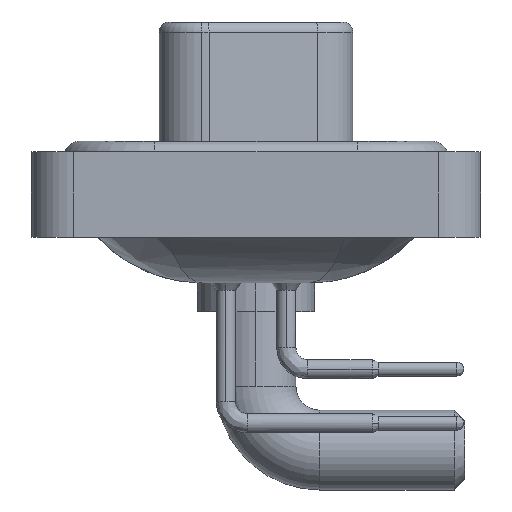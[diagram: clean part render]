
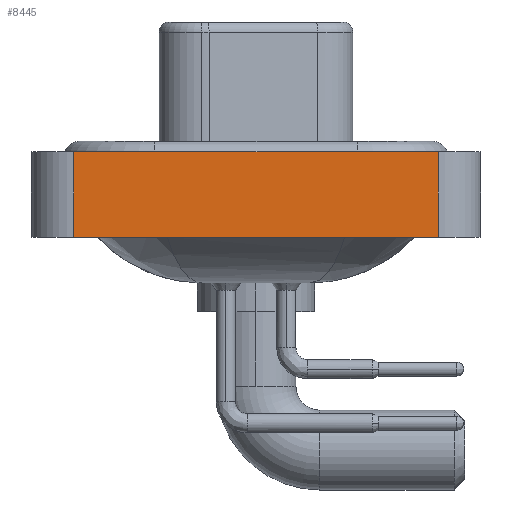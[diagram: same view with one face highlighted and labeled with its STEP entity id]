
A CAD part, left-side view. The second image highlights one B-rep face of the part: STEP entity #8445.
In plain terms, the highlighted planar face has unit normal (-1, 0, 0).
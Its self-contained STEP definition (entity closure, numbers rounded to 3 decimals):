
#60 = CARTESIAN_POINT ( 'NONE',  ( -7.25, 8.55, 0.4 ) ) ;
#461 = VERTEX_POINT ( 'NONE', #8579 ) ;
#969 = CARTESIAN_POINT ( 'NONE',  ( -7.25, -8.55, -3.6 ) ) ;
#2506 = EDGE_LOOP ( 'NONE', ( #13287, #8062, #5538, #6797 ) ) ;
#2616 = VECTOR ( 'NONE', #13395, 1000. ) ;
#3873 = LINE ( 'NONE', #14278, #11997 ) ;
#5166 = FACE_OUTER_BOUND ( 'NONE', #2506, .T. ) ;
#5538 = ORIENTED_EDGE ( 'NONE', *, *, #8697, .F. ) ;
#6797 = ORIENTED_EDGE ( 'NONE', *, *, #21317, .T. ) ;
#7086 = CARTESIAN_POINT ( 'NONE',  ( -7.25, 8.55, -3.6 ) ) ;
#7557 = DIRECTION ( 'NONE',  ( 0., -1., 0. ) ) ;
#8062 = ORIENTED_EDGE ( 'NONE', *, *, #9847, .F. ) ;
#8277 = DIRECTION ( 'NONE',  ( 0., 0., 1. ) ) ;
#8313 = VECTOR ( 'NONE', #21880, 1000. ) ;
#8445 = ADVANCED_FACE ( 'NONE', ( #5166 ), #14073, .T. ) ;
#8579 = CARTESIAN_POINT ( 'NONE',  ( -7.25, -8.55, 0.4 ) ) ;
#8697 = EDGE_CURVE ( 'NONE', #20557, #12375, #11163, .T. ) ;
#9431 = CARTESIAN_POINT ( 'NONE',  ( -7.25, 8.55, -3.6 ) ) ;
#9593 = AXIS2_PLACEMENT_3D ( 'NONE', #21110, #10588, #8277 ) ;
#9847 = EDGE_CURVE ( 'NONE', #12375, #461, #3873, .T. ) ;
#9947 = EDGE_CURVE ( 'NONE', #16285, #461, #20246, .T. ) ;
#10588 = DIRECTION ( 'NONE',  ( -1., 0., 0. ) ) ;
#11163 = LINE ( 'NONE', #9431, #13009 ) ;
#11997 = VECTOR ( 'NONE', #7557, 1000. ) ;
#12375 = VERTEX_POINT ( 'NONE', #60 ) ;
#13009 = VECTOR ( 'NONE', #16471, 1000. ) ;
#13287 = ORIENTED_EDGE ( 'NONE', *, *, #9947, .T. ) ;
#13395 = DIRECTION ( 'NONE',  ( 0., -1., 0. ) ) ;
#14073 = PLANE ( 'NONE',  #9593 ) ;
#14278 = CARTESIAN_POINT ( 'NONE',  ( -7.25, -8.55, 0.4 ) ) ;
#16285 = VERTEX_POINT ( 'NONE', #18890 ) ;
#16471 = DIRECTION ( 'NONE',  ( 0., 0., 1. ) ) ;
#18890 = CARTESIAN_POINT ( 'NONE',  ( -7.25, -8.55, -3.6 ) ) ;
#20246 = LINE ( 'NONE', #969, #8313 ) ;
#20557 = VERTEX_POINT ( 'NONE', #7086 ) ;
#21110 = CARTESIAN_POINT ( 'NONE',  ( -7.25, -8.55, -3.6 ) ) ;
#21317 = EDGE_CURVE ( 'NONE', #20557, #16285, #22172, .T. ) ;
#21880 = DIRECTION ( 'NONE',  ( 0., 0., 1. ) ) ;
#22172 = LINE ( 'NONE', #22511, #2616 ) ;
#22511 = CARTESIAN_POINT ( 'NONE',  ( -7.25, -8.55, -3.6 ) ) ;
